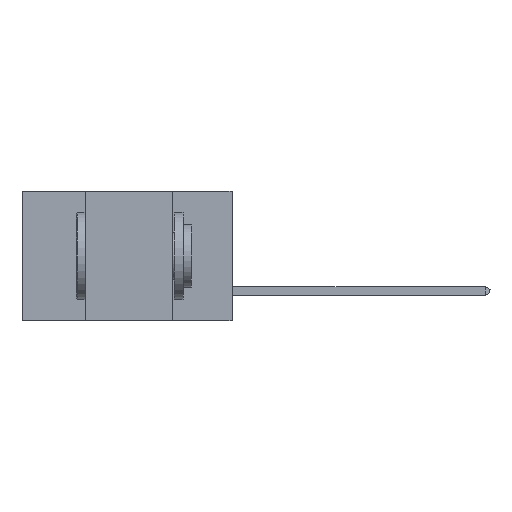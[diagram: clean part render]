
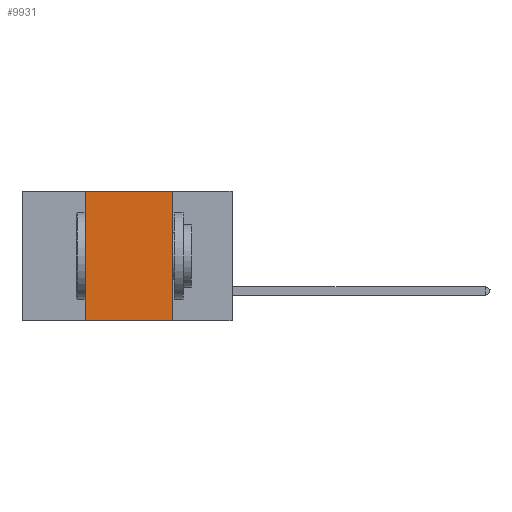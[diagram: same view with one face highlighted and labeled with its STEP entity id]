
A CAD part, left-side view. The second image highlights one B-rep face of the part: STEP entity #9931.
In plain terms, the highlighted planar face has unit normal (-1, 0, 0).
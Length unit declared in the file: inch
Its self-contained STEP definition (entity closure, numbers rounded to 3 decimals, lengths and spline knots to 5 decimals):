
#219 = ORIENTED_EDGE ( 'NONE', *, *, #4731, .T. ) ;
#285 = CARTESIAN_POINT ( 'NONE',  ( 0., 0.6, -0.37 ) ) ;
#2317 = AXIS2_PLACEMENT_3D ( 'NONE', #5093, #9114, #12905 ) ;
#2641 = EDGE_CURVE ( 'NONE', #12263, #5137, #15056, .T. ) ;
#3140 = ORIENTED_EDGE ( 'NONE', *, *, #2641, .F. ) ;
#3715 = VECTOR ( 'NONE', #14504, 39.37008 ) ;
#3745 = CARTESIAN_POINT ( 'NONE',  ( 0., 0.42, -0.37 ) ) ;
#4388 = ORIENTED_EDGE ( 'NONE', *, *, #12414, .F. ) ;
#4731 = EDGE_CURVE ( 'NONE', #12263, #8659, #13962, .T. ) ;
#5093 = CARTESIAN_POINT ( 'NONE',  ( 0., 0.6, 0. ) ) ;
#5137 = VERTEX_POINT ( 'NONE', #12860 ) ;
#5514 = DIRECTION ( 'NONE',  ( 0., -1., 0. ) ) ;
#5669 = DIRECTION ( 'NONE',  ( 0., -1., 0. ) ) ;
#5861 = VERTEX_POINT ( 'NONE', #7521 ) ;
#6111 = ORIENTED_EDGE ( 'NONE', *, *, #17203, .F. ) ;
#6402 = CARTESIAN_POINT ( 'NONE',  ( 0., 0.17, 0. ) ) ;
#6836 = EDGE_LOOP ( 'NONE', ( #6111, #4388, #3140, #219 ) ) ;
#7521 = CARTESIAN_POINT ( 'NONE',  ( 0., 0.17, 0. ) ) ;
#8659 = VERTEX_POINT ( 'NONE', #9913 ) ;
#8943 = CARTESIAN_POINT ( 'NONE',  ( 0., 0.6, 0. ) ) ;
#9006 = CARTESIAN_POINT ( 'NONE',  ( 0., 0.42, 0. ) ) ;
#9114 = DIRECTION ( 'NONE',  ( 1., 0., 0. ) ) ;
#9913 = CARTESIAN_POINT ( 'NONE',  ( 0., 0.17, -0.37 ) ) ;
#9931 = ADVANCED_FACE ( 'NONE', ( #12412 ), #12968, .F. ) ;
#11486 = VECTOR ( 'NONE', #5669, 39.37008 ) ;
#12263 = VERTEX_POINT ( 'NONE', #3745 ) ;
#12317 = LINE ( 'NONE', #6402, #3715 ) ;
#12412 = FACE_OUTER_BOUND ( 'NONE', #6836, .T. ) ;
#12414 = EDGE_CURVE ( 'NONE', #5137, #5861, #15033, .T. ) ;
#12860 = CARTESIAN_POINT ( 'NONE',  ( 0., 0.42, 0. ) ) ;
#12905 = DIRECTION ( 'NONE',  ( 0., 0., -1. ) ) ;
#12968 = PLANE ( 'NONE',  #2317 ) ;
#13962 = LINE ( 'NONE', #285, #16702 ) ;
#14359 = DIRECTION ( 'NONE',  ( 0., 0., 1. ) ) ;
#14504 = DIRECTION ( 'NONE',  ( 0., 0., -1. ) ) ;
#15033 = LINE ( 'NONE', #8943, #11486 ) ;
#15056 = LINE ( 'NONE', #9006, #16339 ) ;
#16339 = VECTOR ( 'NONE', #14359, 39.37008 ) ;
#16702 = VECTOR ( 'NONE', #5514, 39.37008 ) ;
#17203 = EDGE_CURVE ( 'NONE', #5861, #8659, #12317, .T. ) ;
